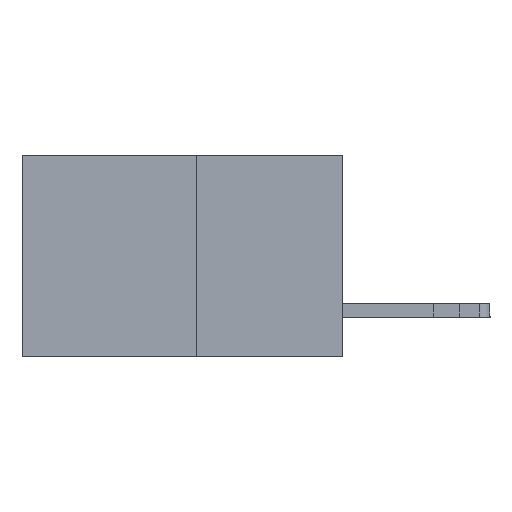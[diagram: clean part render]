
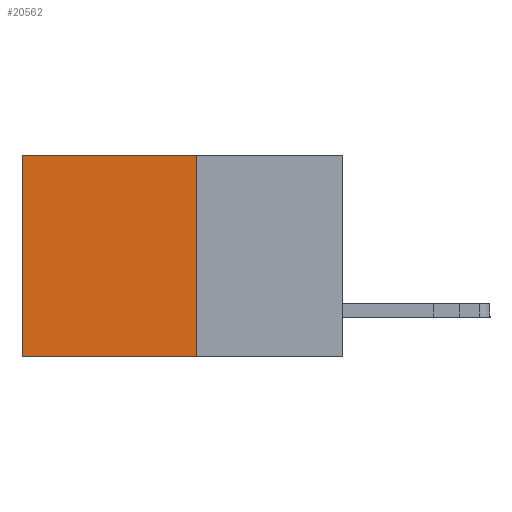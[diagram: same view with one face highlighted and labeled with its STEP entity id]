
A CAD part, left-side view. The second image highlights one B-rep face of the part: STEP entity #20562.
In plain terms, the highlighted planar face has unit normal (-1, 0, 0).
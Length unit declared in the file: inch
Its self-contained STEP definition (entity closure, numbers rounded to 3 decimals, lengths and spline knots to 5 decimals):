
#63 = DIRECTION ( 'NONE',  ( 1., 0., 0. ) ) ;
#384 = CARTESIAN_POINT ( 'NONE',  ( 0.277, 0.27, 0. ) ) ;
#599 = EDGE_CURVE ( 'NONE', #1564, #14562, #17746, .T. ) ;
#1564 = VERTEX_POINT ( 'NONE', #17366 ) ;
#1755 = CARTESIAN_POINT ( 'NONE',  ( 0.277, 0.27, -0.37 ) ) ;
#2395 = EDGE_CURVE ( 'NONE', #17131, #11461, #17077, .T. ) ;
#2697 = LINE ( 'NONE', #18777, #16806 ) ;
#3497 = VECTOR ( 'NONE', #15695, 39.37008 ) ;
#3526 = EDGE_LOOP ( 'NONE', ( #12563, #13115, #18172, #6229 ) ) ;
#3542 = DIRECTION ( 'NONE',  ( 0., 1., 0. ) ) ;
#4708 = VECTOR ( 'NONE', #3542, 39.37008 ) ;
#5192 = CARTESIAN_POINT ( 'NONE',  ( 0.277, 0.59, -0.37 ) ) ;
#6229 = ORIENTED_EDGE ( 'NONE', *, *, #2395, .T. ) ;
#6614 = AXIS2_PLACEMENT_3D ( 'NONE', #1755, #63, #12085 ) ;
#6939 = VECTOR ( 'NONE', #18901, 39.37008 ) ;
#7501 = LINE ( 'NONE', #17180, #6939 ) ;
#8887 = CARTESIAN_POINT ( 'NONE',  ( 0.277, 0.27, 0. ) ) ;
#10384 = PLANE ( 'NONE',  #6614 ) ;
#11461 = VERTEX_POINT ( 'NONE', #21822 ) ;
#12085 = DIRECTION ( 'NONE',  ( 0., 0., -1. ) ) ;
#12563 = ORIENTED_EDGE ( 'NONE', *, *, #20531, .T. ) ;
#13115 = ORIENTED_EDGE ( 'NONE', *, *, #599, .F. ) ;
#14562 = VERTEX_POINT ( 'NONE', #5192 ) ;
#15355 = DIRECTION ( 'NONE',  ( 0., 0., -1. ) ) ;
#15695 = DIRECTION ( 'NONE',  ( 0., 1., 0. ) ) ;
#16806 = VECTOR ( 'NONE', #15355, 39.37008 ) ;
#17077 = LINE ( 'NONE', #8887, #3497 ) ;
#17131 = VERTEX_POINT ( 'NONE', #384 ) ;
#17180 = CARTESIAN_POINT ( 'NONE',  ( 0.277, 0.27, -0.37 ) ) ;
#17366 = CARTESIAN_POINT ( 'NONE',  ( 0.277, 0.27, -0.37 ) ) ;
#17746 = LINE ( 'NONE', #19071, #4708 ) ;
#18172 = ORIENTED_EDGE ( 'NONE', *, *, #21173, .F. ) ;
#18777 = CARTESIAN_POINT ( 'NONE',  ( 0.277, 0.59, -0.37 ) ) ;
#18901 = DIRECTION ( 'NONE',  ( 0., 0., -1. ) ) ;
#19071 = CARTESIAN_POINT ( 'NONE',  ( 0.277, 0.27, -0.37 ) ) ;
#19752 = FACE_OUTER_BOUND ( 'NONE', #3526, .T. ) ;
#20531 = EDGE_CURVE ( 'NONE', #11461, #14562, #2697, .T. ) ;
#20562 = ADVANCED_FACE ( 'NONE', ( #19752 ), #10384, .F. ) ;
#21173 = EDGE_CURVE ( 'NONE', #17131, #1564, #7501, .T. ) ;
#21822 = CARTESIAN_POINT ( 'NONE',  ( 0.277, 0.59, 0. ) ) ;
